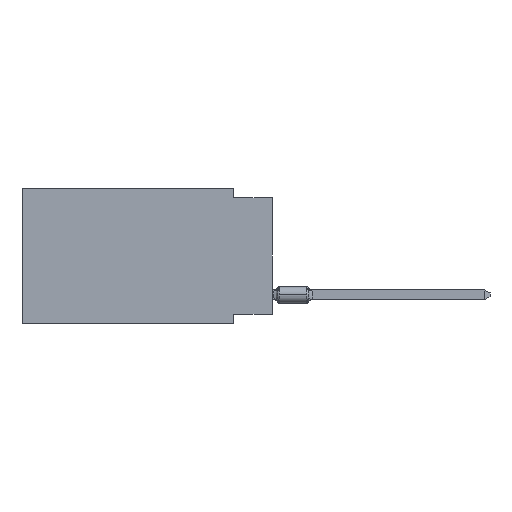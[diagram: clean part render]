
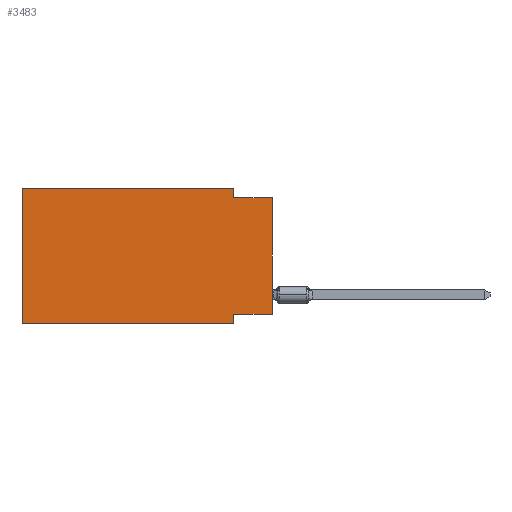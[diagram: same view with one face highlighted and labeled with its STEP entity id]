
A CAD part, left-side view. The second image highlights one B-rep face of the part: STEP entity #3483.
In plain terms, the highlighted planar face has unit normal (-1, 0, 0).
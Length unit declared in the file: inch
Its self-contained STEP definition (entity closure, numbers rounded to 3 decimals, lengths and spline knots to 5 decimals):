
#1291 = CARTESIAN_POINT ( 'NONE',  ( 0., 0.1, -0.325 ) ) ;
#1481 = VECTOR ( 'NONE', #22726, 39.37008 ) ;
#1851 = EDGE_CURVE ( 'NONE', #15789, #5353, #36837, .T. ) ;
#1936 = LINE ( 'NONE', #10823, #28499 ) ;
#2690 = ORIENTED_EDGE ( 'NONE', *, *, #30846, .F. ) ;
#3295 = CARTESIAN_POINT ( 'NONE',  ( 0., 0.1, -0.35 ) ) ;
#3483 = ADVANCED_FACE ( 'NONE', ( #12548 ), #30304, .F. ) ;
#3631 = ORIENTED_EDGE ( 'NONE', *, *, #15042, .F. ) ;
#5353 = VERTEX_POINT ( 'NONE', #15705 ) ;
#5941 = VERTEX_POINT ( 'NONE', #25127 ) ;
#6437 = CARTESIAN_POINT ( 'NONE',  ( 0., 0., 0. ) ) ;
#7145 = DIRECTION ( 'NONE',  ( 0., 1., 0. ) ) ;
#7257 = DIRECTION ( 'NONE',  ( 0., 0., -1. ) ) ;
#7495 = CARTESIAN_POINT ( 'NONE',  ( 0., 0.645, 0. ) ) ;
#8746 = EDGE_CURVE ( 'NONE', #37728, #15789, #1936, .T. ) ;
#9119 = CARTESIAN_POINT ( 'NONE',  ( 0., 0.1, 0. ) ) ;
#9825 = DIRECTION ( 'NONE',  ( 0., 0., -1. ) ) ;
#10823 = CARTESIAN_POINT ( 'NONE',  ( 0., 0., -0.325 ) ) ;
#10948 = CARTESIAN_POINT ( 'NONE',  ( 0., 0.645, -0.35 ) ) ;
#11551 = EDGE_CURVE ( 'NONE', #29980, #37363, #25839, .T. ) ;
#12548 = FACE_OUTER_BOUND ( 'NONE', #25965, .T. ) ;
#12727 = CARTESIAN_POINT ( 'NONE',  ( 0., 0.645, 0. ) ) ;
#12915 = LINE ( 'NONE', #7495, #33652 ) ;
#13307 = DIRECTION ( 'NONE',  ( 0., 0., 1. ) ) ;
#13425 = VECTOR ( 'NONE', #14629, 39.37008 ) ;
#14034 = AXIS2_PLACEMENT_3D ( 'NONE', #12727, #36305, #9825 ) ;
#14153 = LINE ( 'NONE', #20712, #25272 ) ;
#14244 = CARTESIAN_POINT ( 'NONE',  ( 0., 0., -0.025 ) ) ;
#14629 = DIRECTION ( 'NONE',  ( 0., -1., 0. ) ) ;
#14901 = ORIENTED_EDGE ( 'NONE', *, *, #1851, .F. ) ;
#15042 = EDGE_CURVE ( 'NONE', #19567, #29980, #29590, .T. ) ;
#15146 = ORIENTED_EDGE ( 'NONE', *, *, #24349, .T. ) ;
#15705 = CARTESIAN_POINT ( 'NONE',  ( 0., 0.1, -0.35 ) ) ;
#15789 = VERTEX_POINT ( 'NONE', #1291 ) ;
#16000 = ORIENTED_EDGE ( 'NONE', *, *, #11551, .F. ) ;
#16739 = VERTEX_POINT ( 'NONE', #18428 ) ;
#16759 = VECTOR ( 'NONE', #24336, 39.37008 ) ;
#18428 = CARTESIAN_POINT ( 'NONE',  ( 0., 0.645, -0.35 ) ) ;
#19567 = VERTEX_POINT ( 'NONE', #29862 ) ;
#19734 = CARTESIAN_POINT ( 'NONE',  ( 0., 0., -0.025 ) ) ;
#19851 = EDGE_CURVE ( 'NONE', #16739, #5941, #12915, .T. ) ;
#20546 = DIRECTION ( 'NONE',  ( 0., 0., 1. ) ) ;
#20712 = CARTESIAN_POINT ( 'NONE',  ( 0., 0.645, 0. ) ) ;
#22726 = DIRECTION ( 'NONE',  ( 0., -1., 0. ) ) ;
#22908 = LINE ( 'NONE', #10948, #1481 ) ;
#23517 = VECTOR ( 'NONE', #7257, 39.37008 ) ;
#24336 = DIRECTION ( 'NONE',  ( 0., 0., -1. ) ) ;
#24349 = EDGE_CURVE ( 'NONE', #16739, #5353, #22908, .T. ) ;
#24398 = ORIENTED_EDGE ( 'NONE', *, *, #19851, .F. ) ;
#25127 = CARTESIAN_POINT ( 'NONE',  ( 0., 0.645, 0. ) ) ;
#25272 = VECTOR ( 'NONE', #26524, 39.37008 ) ;
#25301 = CARTESIAN_POINT ( 'NONE',  ( 0., 0., -0.325 ) ) ;
#25839 = LINE ( 'NONE', #14244, #13425 ) ;
#25965 = EDGE_LOOP ( 'NONE', ( #36164, #16000, #3631, #2690, #24398, #15146, #14901, #30571 ) ) ;
#26524 = DIRECTION ( 'NONE',  ( 0., -1., 0. ) ) ;
#28499 = VECTOR ( 'NONE', #7145, 39.37008 ) ;
#29590 = LINE ( 'NONE', #9119, #16759 ) ;
#29862 = CARTESIAN_POINT ( 'NONE',  ( 0., 0.1, 0. ) ) ;
#29980 = VERTEX_POINT ( 'NONE', #30724 ) ;
#30304 = PLANE ( 'NONE',  #14034 ) ;
#30571 = ORIENTED_EDGE ( 'NONE', *, *, #8746, .F. ) ;
#30724 = CARTESIAN_POINT ( 'NONE',  ( 0., 0.1, -0.025 ) ) ;
#30846 = EDGE_CURVE ( 'NONE', #5941, #19567, #14153, .T. ) ;
#31369 = VECTOR ( 'NONE', #20546, 39.37008 ) ;
#33652 = VECTOR ( 'NONE', #13307, 39.37008 ) ;
#35638 = LINE ( 'NONE', #6437, #31369 ) ;
#35734 = EDGE_CURVE ( 'NONE', #37728, #37363, #35638, .T. ) ;
#36164 = ORIENTED_EDGE ( 'NONE', *, *, #35734, .T. ) ;
#36305 = DIRECTION ( 'NONE',  ( 1., 0., 0. ) ) ;
#36837 = LINE ( 'NONE', #3295, #23517 ) ;
#37363 = VERTEX_POINT ( 'NONE', #19734 ) ;
#37728 = VERTEX_POINT ( 'NONE', #25301 ) ;
